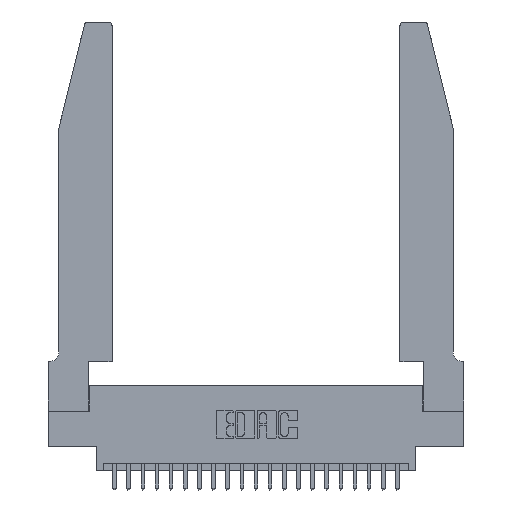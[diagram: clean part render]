
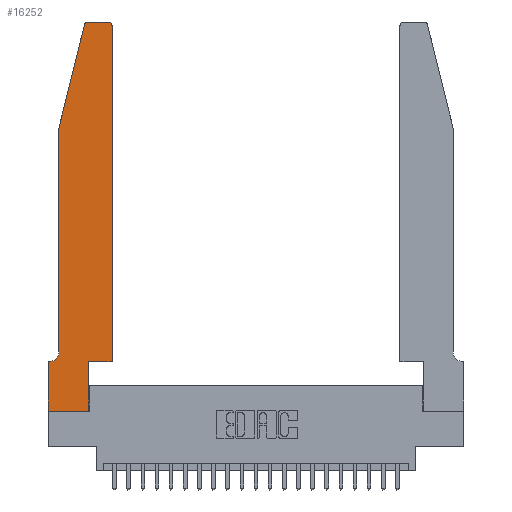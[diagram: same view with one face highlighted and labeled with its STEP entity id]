
A CAD part, top view. The second image highlights one B-rep face of the part: STEP entity #16252.
In plain terms, the highlighted planar face has unit normal (0, 0, 1).
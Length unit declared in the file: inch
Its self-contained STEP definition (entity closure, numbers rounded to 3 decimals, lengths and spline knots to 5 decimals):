
#1459 = DIRECTION ( 'NONE',  ( 0., -1., 0. ) ) ;
#1531 = VERTEX_POINT ( 'NONE', #5863 ) ;
#1614 = LINE ( 'NONE', #16435, #16027 ) ;
#1682 = DIRECTION ( 'NONE',  ( -1., 0., 0. ) ) ;
#1692 = VECTOR ( 'NONE', #10872, 39.37008 ) ;
#1913 = CIRCLE ( 'NONE', #9398, 0.07 ) ;
#1981 = ORIENTED_EDGE ( 'NONE', *, *, #11610, .T. ) ;
#2017 = DIRECTION ( 'NONE',  ( 0., 1., 0. ) ) ;
#2055 = ORIENTED_EDGE ( 'NONE', *, *, #4370, .T. ) ;
#2436 = ORIENTED_EDGE ( 'NONE', *, *, #11721, .T. ) ;
#2586 = ORIENTED_EDGE ( 'NONE', *, *, #17055, .T. ) ;
#2761 = LINE ( 'NONE', #24060, #18344 ) ;
#2992 = ORIENTED_EDGE ( 'NONE', *, *, #11747, .T. ) ;
#3862 = VECTOR ( 'NONE', #17871, 39.37008 ) ;
#4370 = EDGE_CURVE ( 'NONE', #9851, #17089, #14670, .T. ) ;
#4377 = LINE ( 'NONE', #6819, #19303 ) ;
#4468 = LINE ( 'NONE', #19733, #3862 ) ;
#4510 = EDGE_CURVE ( 'NONE', #1531, #21910, #7985, .T. ) ;
#4839 = CARTESIAN_POINT ( 'NONE',  ( 0.4205, 2.72, 0.37 ) ) ;
#5362 = ORIENTED_EDGE ( 'NONE', *, *, #7220, .T. ) ;
#5863 = CARTESIAN_POINT ( 'NONE',  ( 0., 0.35, 0.37 ) ) ;
#5872 = CARTESIAN_POINT ( 'NONE',  ( 0.4505, 0.35, 0.37 ) ) ;
#6092 = CARTESIAN_POINT ( 'NONE',  ( 0.0755, 2., 0.37 ) ) ;
#6102 = VERTEX_POINT ( 'NONE', #5872 ) ;
#6113 = EDGE_CURVE ( 'NONE', #8562, #1531, #22964, .T. ) ;
#6774 = DIRECTION ( 'NONE',  ( 1., 0., 0. ) ) ;
#6819 = CARTESIAN_POINT ( 'NONE',  ( 0.0755, 2., 0.37 ) ) ;
#6865 = CARTESIAN_POINT ( 'NONE',  ( 0.284, 2.72, 0.37 ) ) ;
#6913 = EDGE_CURVE ( 'NONE', #10134, #8562, #1913, .T. ) ;
#7220 = EDGE_CURVE ( 'NONE', #22961, #10134, #1614, .T. ) ;
#7592 = EDGE_LOOP ( 'NONE', ( #10686, #22359, #2992, #5362, #8687, #15328, #19449, #2436, #2586, #1981, #23366, #2055 ) ) ;
#7826 = VERTEX_POINT ( 'NONE', #10972 ) ;
#7959 = LINE ( 'NONE', #9807, #17259 ) ;
#7985 = LINE ( 'NONE', #20039, #1692 ) ;
#8562 = VERTEX_POINT ( 'NONE', #11573 ) ;
#8650 = LINE ( 'NONE', #13326, #13585 ) ;
#8687 = ORIENTED_EDGE ( 'NONE', *, *, #6913, .T. ) ;
#8762 = DIRECTION ( 'NONE',  ( 1., 0., 0. ) ) ;
#8847 = DIRECTION ( 'NONE',  ( 0., 0., 1. ) ) ;
#9304 = CARTESIAN_POINT ( 'NONE',  ( 0.0755, 0.42, 0.37 ) ) ;
#9398 = AXIS2_PLACEMENT_3D ( 'NONE', #10832, #23753, #12690 ) ;
#9807 = CARTESIAN_POINT ( 'NONE',  ( 0.4505, 0.35, 0.37 ) ) ;
#9851 = VERTEX_POINT ( 'NONE', #19326 ) ;
#10134 = VERTEX_POINT ( 'NONE', #9304 ) ;
#10686 = ORIENTED_EDGE ( 'NONE', *, *, #22128, .T. ) ;
#10832 = CARTESIAN_POINT ( 'NONE',  ( 0.0055, 0.42, 0.37 ) ) ;
#10872 = DIRECTION ( 'NONE',  ( 0., -1., 0. ) ) ;
#10972 = CARTESIAN_POINT ( 'NONE',  ( 0.2865, 0., 0.37 ) ) ;
#11521 = CARTESIAN_POINT ( 'NONE',  ( 0.0755, 0.35, 0.37 ) ) ;
#11573 = CARTESIAN_POINT ( 'NONE',  ( 0.0055, 0.35, 0.37 ) ) ;
#11610 = EDGE_CURVE ( 'NONE', #14037, #6102, #7959, .T. ) ;
#11670 = VERTEX_POINT ( 'NONE', #21125 ) ;
#11721 = EDGE_CURVE ( 'NONE', #21910, #7826, #4468, .T. ) ;
#11747 = EDGE_CURVE ( 'NONE', #16448, #22961, #4377, .T. ) ;
#11759 = CIRCLE ( 'NONE', #21372, 0.03 ) ;
#12690 = DIRECTION ( 'NONE',  ( -1., 0., 0. ) ) ;
#13028 = CARTESIAN_POINT ( 'NONE',  ( 0.4205, 2.75, 0.37 ) ) ;
#13326 = CARTESIAN_POINT ( 'NONE',  ( 0.4505, 0.35, 0.37 ) ) ;
#13585 = VECTOR ( 'NONE', #2017, 39.37008 ) ;
#13712 = VECTOR ( 'NONE', #18934, 39.37008 ) ;
#14037 = VERTEX_POINT ( 'NONE', #20862 ) ;
#14355 = PLANE ( 'NONE',  #16663 ) ;
#14670 = CIRCLE ( 'NONE', #15806, 0.03 ) ;
#14826 = CARTESIAN_POINT ( 'NONE',  ( 0.2865, 0.35, 0.37 ) ) ;
#15328 = ORIENTED_EDGE ( 'NONE', *, *, #6113, .T. ) ;
#15806 = AXIS2_PLACEMENT_3D ( 'NONE', #4839, #17931, #6774 ) ;
#16027 = VECTOR ( 'NONE', #1459, 39.37008 ) ;
#16252 = ADVANCED_FACE ( 'NONE', ( #18353 ), #14355, .T. ) ;
#16435 = CARTESIAN_POINT ( 'NONE',  ( 0.0755, 2., 0.37 ) ) ;
#16448 = VERTEX_POINT ( 'NONE', #16787 ) ;
#16663 = AXIS2_PLACEMENT_3D ( 'NONE', #19969, #8847, #21790 ) ;
#16787 = CARTESIAN_POINT ( 'NONE',  ( 0.25487, 2.72718, 0.37 ) ) ;
#16852 = VECTOR ( 'NONE', #18576, 39.37008 ) ;
#17055 = EDGE_CURVE ( 'NONE', #7826, #14037, #21748, .T. ) ;
#17089 = VERTEX_POINT ( 'NONE', #13028 ) ;
#17251 = DIRECTION ( 'NONE',  ( 1., 0., 0. ) ) ;
#17259 = VECTOR ( 'NONE', #17251, 39.37008 ) ;
#17871 = DIRECTION ( 'NONE',  ( 1., 0., 0. ) ) ;
#17931 = DIRECTION ( 'NONE',  ( 0., 0., 1. ) ) ;
#18344 = VECTOR ( 'NONE', #1682, 39.37008 ) ;
#18353 = FACE_OUTER_BOUND ( 'NONE', #7592, .T. ) ;
#18576 = DIRECTION ( 'NONE',  ( 0., 1., 0. ) ) ;
#18934 = DIRECTION ( 'NONE',  ( -1., 0., 0. ) ) ;
#19092 = EDGE_CURVE ( 'NONE', #6102, #9851, #8650, .T. ) ;
#19303 = VECTOR ( 'NONE', #21674, 39.37008 ) ;
#19326 = CARTESIAN_POINT ( 'NONE',  ( 0.4505, 2.72, 0.37 ) ) ;
#19449 = ORIENTED_EDGE ( 'NONE', *, *, #4510, .T. ) ;
#19733 = CARTESIAN_POINT ( 'NONE',  ( 0., 0., 0.37 ) ) ;
#19893 = DIRECTION ( 'NONE',  ( 0., 0., 1. ) ) ;
#19969 = CARTESIAN_POINT ( 'NONE',  ( 0., 0.35, 0.37 ) ) ;
#20039 = CARTESIAN_POINT ( 'NONE',  ( 0., 0., 0.37 ) ) ;
#20862 = CARTESIAN_POINT ( 'NONE',  ( 0.2865, 0.35, 0.37 ) ) ;
#21085 = EDGE_CURVE ( 'NONE', #11670, #16448, #11759, .T. ) ;
#21125 = CARTESIAN_POINT ( 'NONE',  ( 0.284, 2.75, 0.37 ) ) ;
#21372 = AXIS2_PLACEMENT_3D ( 'NONE', #6865, #19893, #8762 ) ;
#21581 = CARTESIAN_POINT ( 'NONE',  ( 0., 0., 0.37 ) ) ;
#21674 = DIRECTION ( 'NONE',  ( -0.239, -0.971, 0. ) ) ;
#21748 = LINE ( 'NONE', #14826, #16852 ) ;
#21790 = DIRECTION ( 'NONE',  ( 1., 0., 0. ) ) ;
#21910 = VERTEX_POINT ( 'NONE', #21581 ) ;
#22128 = EDGE_CURVE ( 'NONE', #17089, #11670, #2761, .T. ) ;
#22359 = ORIENTED_EDGE ( 'NONE', *, *, #21085, .T. ) ;
#22961 = VERTEX_POINT ( 'NONE', #6092 ) ;
#22964 = LINE ( 'NONE', #11521, #13712 ) ;
#23366 = ORIENTED_EDGE ( 'NONE', *, *, #19092, .T. ) ;
#23753 = DIRECTION ( 'NONE',  ( 0., 0., -1. ) ) ;
#24060 = CARTESIAN_POINT ( 'NONE',  ( 0.2605, 2.75, 0.37 ) ) ;
